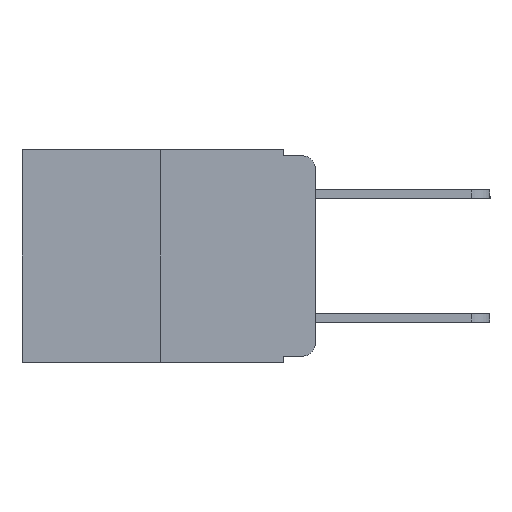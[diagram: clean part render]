
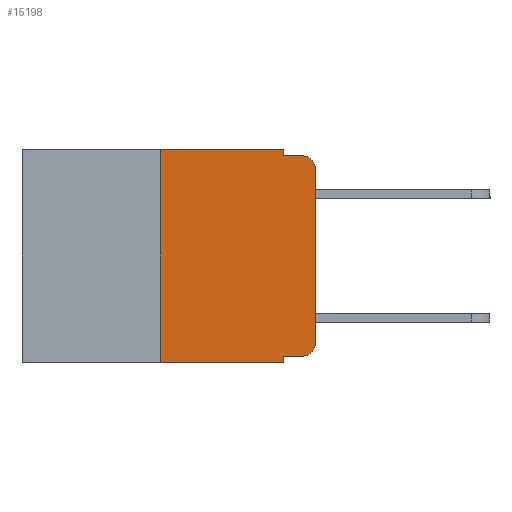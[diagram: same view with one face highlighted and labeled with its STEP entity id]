
A CAD part, left-side view. The second image highlights one B-rep face of the part: STEP entity #15198.
In plain terms, the highlighted planar face has unit normal (-1, 0, 0).
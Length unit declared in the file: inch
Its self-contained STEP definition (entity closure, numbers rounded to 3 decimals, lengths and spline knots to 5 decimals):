
#66 = DIRECTION ( 'NONE',  ( 0., -1., 0. ) ) ;
#72 = VERTEX_POINT ( 'NONE', #18230 ) ;
#79 = EDGE_CURVE ( 'NONE', #13420, #8433, #18593, .T. ) ;
#379 = VECTOR ( 'NONE', #66, 39.37008 ) ;
#411 = ORIENTED_EDGE ( 'NONE', *, *, #11099, .F. ) ;
#626 = VERTEX_POINT ( 'NONE', #18461 ) ;
#863 = LINE ( 'NONE', #13132, #4888 ) ;
#1076 = EDGE_CURVE ( 'NONE', #1657, #3997, #14223, .T. ) ;
#1132 = ORIENTED_EDGE ( 'NONE', *, *, #1076, .T. ) ;
#1411 = EDGE_CURVE ( 'NONE', #3997, #5728, #3316, .T. ) ;
#1625 = EDGE_CURVE ( 'NONE', #72, #13420, #15708, .T. ) ;
#1634 = ORIENTED_EDGE ( 'NONE', *, *, #6982, .T. ) ;
#1657 = VERTEX_POINT ( 'NONE', #5825 ) ;
#2261 = DIRECTION ( 'NONE',  ( 0., -1., 0. ) ) ;
#2403 = EDGE_LOOP ( 'NONE', ( #8689, #5414, #13681, #3398, #3701, #411, #1634, #11917, #4231, #1132 ) ) ;
#2598 = VECTOR ( 'NONE', #16485, 39.37008 ) ;
#3316 = LINE ( 'NONE', #7470, #18744 ) ;
#3385 = CARTESIAN_POINT ( 'NONE',  ( 0., 0.051, 0. ) ) ;
#3398 = ORIENTED_EDGE ( 'NONE', *, *, #79, .F. ) ;
#3575 = VECTOR ( 'NONE', #12873, 39.37008 ) ;
#3701 = ORIENTED_EDGE ( 'NONE', *, *, #1625, .F. ) ;
#3997 = VERTEX_POINT ( 'NONE', #12527 ) ;
#4033 = VERTEX_POINT ( 'NONE', #15774 ) ;
#4231 = ORIENTED_EDGE ( 'NONE', *, *, #17493, .T. ) ;
#4314 = AXIS2_PLACEMENT_3D ( 'NONE', #8810, #16841, #16822 ) ;
#4319 = VECTOR ( 'NONE', #19073, 39.37008 ) ;
#4888 = VECTOR ( 'NONE', #5500, 39.37008 ) ;
#4925 = CARTESIAN_POINT ( 'NONE',  ( 0., 0.051, -0.01 ) ) ;
#4970 = LINE ( 'NONE', #10059, #379 ) ;
#4984 = AXIS2_PLACEMENT_3D ( 'NONE', #16047, #18851, #10499 ) ;
#5414 = ORIENTED_EDGE ( 'NONE', *, *, #14069, .T. ) ;
#5500 = DIRECTION ( 'NONE',  ( 0., 0., -1. ) ) ;
#5728 = VERTEX_POINT ( 'NONE', #18231 ) ;
#5825 = CARTESIAN_POINT ( 'NONE',  ( 0., 0.02, -0.333 ) ) ;
#6582 = DIRECTION ( 'NONE',  ( -1., 0., 0. ) ) ;
#6982 = EDGE_CURVE ( 'NONE', #11196, #626, #16332, .T. ) ;
#7088 = LINE ( 'NONE', #9654, #18147 ) ;
#7470 = CARTESIAN_POINT ( 'NONE',  ( 0., 0., 0. ) ) ;
#8110 = DIRECTION ( 'NONE',  ( 0., 0., 1. ) ) ;
#8230 = EDGE_CURVE ( 'NONE', #8433, #4033, #13062, .T. ) ;
#8433 = VERTEX_POINT ( 'NONE', #4925 ) ;
#8497 = CIRCLE ( 'NONE', #11434, 0.02 ) ;
#8630 = CARTESIAN_POINT ( 'NONE',  ( 0., 0.473, 0. ) ) ;
#8689 = ORIENTED_EDGE ( 'NONE', *, *, #1411, .T. ) ;
#8810 = CARTESIAN_POINT ( 'NONE',  ( 0., 0.02, -0.313 ) ) ;
#9654 = CARTESIAN_POINT ( 'NONE',  ( 0., 0.25, 0. ) ) ;
#10059 = CARTESIAN_POINT ( 'NONE',  ( 0., 0.051, -0.333 ) ) ;
#10499 = DIRECTION ( 'NONE',  ( 0., 0., -1. ) ) ;
#10763 = VERTEX_POINT ( 'NONE', #16011 ) ;
#11099 = EDGE_CURVE ( 'NONE', #11196, #72, #7088, .T. ) ;
#11196 = VERTEX_POINT ( 'NONE', #14100 ) ;
#11434 = AXIS2_PLACEMENT_3D ( 'NONE', #15361, #6582, #16742 ) ;
#11917 = ORIENTED_EDGE ( 'NONE', *, *, #18151, .F. ) ;
#12527 = CARTESIAN_POINT ( 'NONE',  ( 0., 0., -0.313 ) ) ;
#12813 = FACE_OUTER_BOUND ( 'NONE', #2403, .T. ) ;
#12873 = DIRECTION ( 'NONE',  ( 0., -1., 0. ) ) ;
#13062 = LINE ( 'NONE', #13585, #4319 ) ;
#13132 = CARTESIAN_POINT ( 'NONE',  ( 0., 0.051, 0. ) ) ;
#13306 = PLANE ( 'NONE',  #4984 ) ;
#13420 = VERTEX_POINT ( 'NONE', #3385 ) ;
#13585 = CARTESIAN_POINT ( 'NONE',  ( 0., 0.051, -0.01 ) ) ;
#13681 = ORIENTED_EDGE ( 'NONE', *, *, #8230, .F. ) ;
#14069 = EDGE_CURVE ( 'NONE', #5728, #4033, #8497, .T. ) ;
#14100 = CARTESIAN_POINT ( 'NONE',  ( 0., 0.25, -0.343 ) ) ;
#14223 = CIRCLE ( 'NONE', #4314, 0.02 ) ;
#15198 = ADVANCED_FACE ( 'NONE', ( #12813 ), #13306, .F. ) ;
#15361 = CARTESIAN_POINT ( 'NONE',  ( 0., 0.02, -0.03 ) ) ;
#15708 = LINE ( 'NONE', #8630, #3575 ) ;
#15774 = CARTESIAN_POINT ( 'NONE',  ( 0., 0.02, -0.01 ) ) ;
#15905 = VECTOR ( 'NONE', #2261, 39.37008 ) ;
#15975 = CARTESIAN_POINT ( 'NONE',  ( 0., 0.473, -0.343 ) ) ;
#16011 = CARTESIAN_POINT ( 'NONE',  ( 0., 0.051, -0.333 ) ) ;
#16047 = CARTESIAN_POINT ( 'NONE',  ( 0., 0.473, 0. ) ) ;
#16332 = LINE ( 'NONE', #15975, #15905 ) ;
#16421 = CARTESIAN_POINT ( 'NONE',  ( 0., 0.051, 0. ) ) ;
#16485 = DIRECTION ( 'NONE',  ( 0., 0., -1. ) ) ;
#16742 = DIRECTION ( 'NONE',  ( 0., 0., -1. ) ) ;
#16822 = DIRECTION ( 'NONE',  ( 0., 0., -1. ) ) ;
#16841 = DIRECTION ( 'NONE',  ( -1., 0., 0. ) ) ;
#17465 = DIRECTION ( 'NONE',  ( 0., 0., 1. ) ) ;
#17493 = EDGE_CURVE ( 'NONE', #10763, #1657, #4970, .T. ) ;
#18147 = VECTOR ( 'NONE', #8110, 39.37008 ) ;
#18151 = EDGE_CURVE ( 'NONE', #10763, #626, #863, .T. ) ;
#18230 = CARTESIAN_POINT ( 'NONE',  ( 0., 0.25, 0. ) ) ;
#18231 = CARTESIAN_POINT ( 'NONE',  ( 0., 0., -0.03 ) ) ;
#18461 = CARTESIAN_POINT ( 'NONE',  ( 0., 0.051, -0.343 ) ) ;
#18593 = LINE ( 'NONE', #16421, #2598 ) ;
#18744 = VECTOR ( 'NONE', #17465, 39.37008 ) ;
#18851 = DIRECTION ( 'NONE',  ( 1., 0., 0. ) ) ;
#19073 = DIRECTION ( 'NONE',  ( 0., -1., 0. ) ) ;
